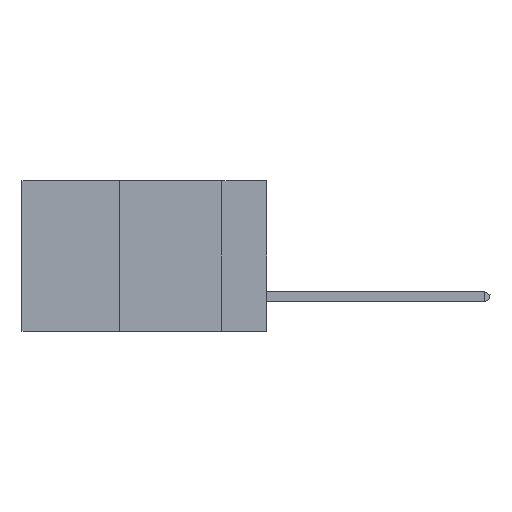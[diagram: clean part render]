
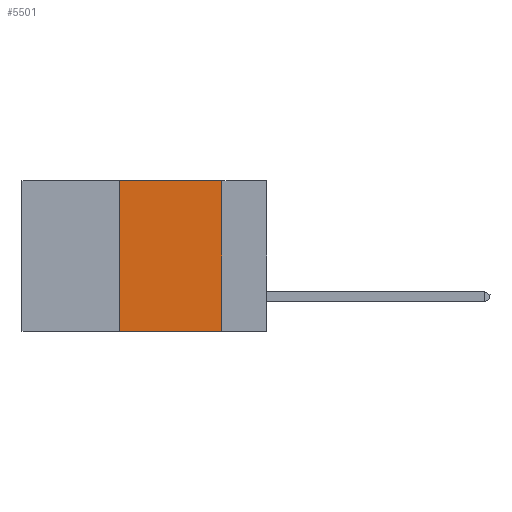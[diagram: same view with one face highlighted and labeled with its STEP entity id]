
A CAD part, left-side view. The second image highlights one B-rep face of the part: STEP entity #5501.
In plain terms, the highlighted planar face has unit normal (-1, 0, 0).
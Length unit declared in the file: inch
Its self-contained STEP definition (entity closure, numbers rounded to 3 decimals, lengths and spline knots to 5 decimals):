
#312 = ORIENTED_EDGE ( 'NONE', *, *, #7161, .T. ) ;
#359 = AXIS2_PLACEMENT_3D ( 'NONE', #5094, #3828, #11889 ) ;
#493 = LINE ( 'NONE', #3519, #7303 ) ;
#1181 = LINE ( 'NONE', #5229, #8587 ) ;
#1434 = VECTOR ( 'NONE', #11733, 39.37008 ) ;
#1495 = CARTESIAN_POINT ( 'NONE',  ( 0., 0.36, 0. ) ) ;
#1766 = VERTEX_POINT ( 'NONE', #9964 ) ;
#2032 = VERTEX_POINT ( 'NONE', #9573 ) ;
#2926 = LINE ( 'NONE', #12908, #1434 ) ;
#2960 = FACE_OUTER_BOUND ( 'NONE', #12537, .T. ) ;
#3519 = CARTESIAN_POINT ( 'NONE',  ( 0., 0.36, 0. ) ) ;
#3719 = EDGE_CURVE ( 'NONE', #11818, #11412, #493, .T. ) ;
#3828 = DIRECTION ( 'NONE',  ( 1., 0., 0. ) ) ;
#4235 = ORIENTED_EDGE ( 'NONE', *, *, #5591, .F. ) ;
#5094 = CARTESIAN_POINT ( 'NONE',  ( 0., 0.6, 0. ) ) ;
#5229 = CARTESIAN_POINT ( 'NONE',  ( 0., 0.6, 0. ) ) ;
#5288 = CARTESIAN_POINT ( 'NONE',  ( 0., 0.11, 0. ) ) ;
#5501 = ADVANCED_FACE ( 'NONE', ( #2960 ), #12876, .F. ) ;
#5591 = EDGE_CURVE ( 'NONE', #2032, #1766, #8373, .T. ) ;
#5774 = ORIENTED_EDGE ( 'NONE', *, *, #3719, .F. ) ;
#6045 = VECTOR ( 'NONE', #9322, 39.37008 ) ;
#6433 = CARTESIAN_POINT ( 'NONE',  ( 0., 0.36, -0.37 ) ) ;
#6674 = EDGE_CURVE ( 'NONE', #11412, #2032, #1181, .T. ) ;
#6920 = ORIENTED_EDGE ( 'NONE', *, *, #6674, .F. ) ;
#7161 = EDGE_CURVE ( 'NONE', #11818, #1766, #2926, .T. ) ;
#7303 = VECTOR ( 'NONE', #11594, 39.37008 ) ;
#8252 = DIRECTION ( 'NONE',  ( 0., -1., 0. ) ) ;
#8373 = LINE ( 'NONE', #5288, #6045 ) ;
#8587 = VECTOR ( 'NONE', #8252, 39.37008 ) ;
#9322 = DIRECTION ( 'NONE',  ( 0., 0., -1. ) ) ;
#9573 = CARTESIAN_POINT ( 'NONE',  ( 0., 0.11, 0. ) ) ;
#9964 = CARTESIAN_POINT ( 'NONE',  ( 0., 0.11, -0.37 ) ) ;
#11412 = VERTEX_POINT ( 'NONE', #1495 ) ;
#11594 = DIRECTION ( 'NONE',  ( 0., 0., 1. ) ) ;
#11733 = DIRECTION ( 'NONE',  ( 0., -1., 0. ) ) ;
#11818 = VERTEX_POINT ( 'NONE', #6433 ) ;
#11889 = DIRECTION ( 'NONE',  ( 0., 0., -1. ) ) ;
#12537 = EDGE_LOOP ( 'NONE', ( #4235, #6920, #5774, #312 ) ) ;
#12876 = PLANE ( 'NONE',  #359 ) ;
#12908 = CARTESIAN_POINT ( 'NONE',  ( 0., 0.6, -0.37 ) ) ;
